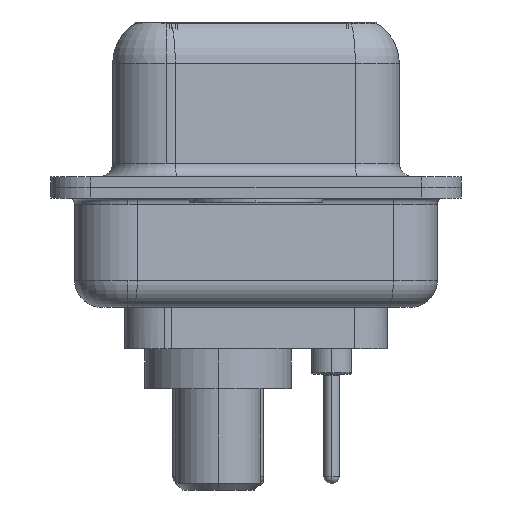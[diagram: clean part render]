
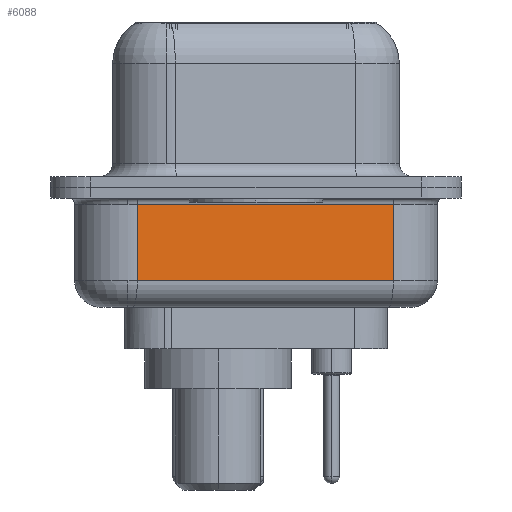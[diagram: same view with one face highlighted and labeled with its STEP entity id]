
A CAD part, left-side view. The second image highlights one B-rep face of the part: STEP entity #6088.
In plain terms, the highlighted planar face has unit normal (-0.985, -0.174, 0).
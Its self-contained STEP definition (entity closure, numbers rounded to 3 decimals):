
#995 = LINE ( 'NONE', #28250, #22098 ) ;
#1213 = VECTOR ( 'NONE', #11646, 1000. ) ;
#1231 = CARTESIAN_POINT ( 'NONE',  ( 2.93, 4.453, -4.5 ) ) ;
#1400 = VERTEX_POINT ( 'NONE', #5974 ) ;
#2027 = CARTESIAN_POINT ( 'NONE',  ( 2.93, 4.453, -3.5 ) ) ;
#2169 = ORIENTED_EDGE ( 'NONE', *, *, #29522, .T. ) ;
#2339 = VECTOR ( 'NONE', #16895, 1000. ) ;
#5902 = CARTESIAN_POINT ( 'NONE',  ( 4.623, -5.147, -3.5 ) ) ;
#5974 = CARTESIAN_POINT ( 'NONE',  ( 2.93, 4.453, -0.65 ) ) ;
#6071 = DIRECTION ( 'NONE',  ( -0.174, 0.985, 0. ) ) ;
#6088 = ADVANCED_FACE ( 'NONE', ( #10024 ), #30742, .F. ) ;
#6138 = ORIENTED_EDGE ( 'NONE', *, *, #26327, .T. ) ;
#6883 = EDGE_CURVE ( 'NONE', #24473, #17131, #17644, .T. ) ;
#8720 = DIRECTION ( 'NONE',  ( -0.174, 0.985, 0. ) ) ;
#9587 = VECTOR ( 'NONE', #29843, 1000. ) ;
#10024 = FACE_OUTER_BOUND ( 'NONE', #25505, .T. ) ;
#11013 = DIRECTION ( 'NONE',  ( 0.985, 0.174, 0. ) ) ;
#11646 = DIRECTION ( 'NONE',  ( 0., 0., 1. ) ) ;
#12595 = ORIENTED_EDGE ( 'NONE', *, *, #16585, .F. ) ;
#14252 = LINE ( 'NONE', #18704, #1213 ) ;
#16585 = EDGE_CURVE ( 'NONE', #25057, #1400, #14252, .T. ) ;
#16895 = DIRECTION ( 'NONE',  ( 0.174, -0.985, 0. ) ) ;
#17131 = VERTEX_POINT ( 'NONE', #20367 ) ;
#17644 = LINE ( 'NONE', #27376, #9587 ) ;
#18704 = CARTESIAN_POINT ( 'NONE',  ( 2.93, 4.453, -4.5 ) ) ;
#20367 = CARTESIAN_POINT ( 'NONE',  ( 4.623, -5.147, -0.65 ) ) ;
#22098 = VECTOR ( 'NONE', #8720, 1000. ) ;
#24473 = VERTEX_POINT ( 'NONE', #5902 ) ;
#25057 = VERTEX_POINT ( 'NONE', #30127 ) ;
#25505 = EDGE_LOOP ( 'NONE', ( #12595, #2169, #31520, #6138 ) ) ;
#25987 = AXIS2_PLACEMENT_3D ( 'NONE', #1231, #11013, #6071 ) ;
#26327 = EDGE_CURVE ( 'NONE', #17131, #1400, #995, .T. ) ;
#27376 = CARTESIAN_POINT ( 'NONE',  ( 4.623, -5.147, -4.5 ) ) ;
#28250 = CARTESIAN_POINT ( 'NONE',  ( 2.93, 4.453, -0.65 ) ) ;
#29522 = EDGE_CURVE ( 'NONE', #25057, #24473, #29989, .T. ) ;
#29843 = DIRECTION ( 'NONE',  ( 0., 0., 1. ) ) ;
#29989 = LINE ( 'NONE', #2027, #2339 ) ;
#30127 = CARTESIAN_POINT ( 'NONE',  ( 2.93, 4.453, -3.5 ) ) ;
#30742 = PLANE ( 'NONE',  #25987 ) ;
#31520 = ORIENTED_EDGE ( 'NONE', *, *, #6883, .T. ) ;
